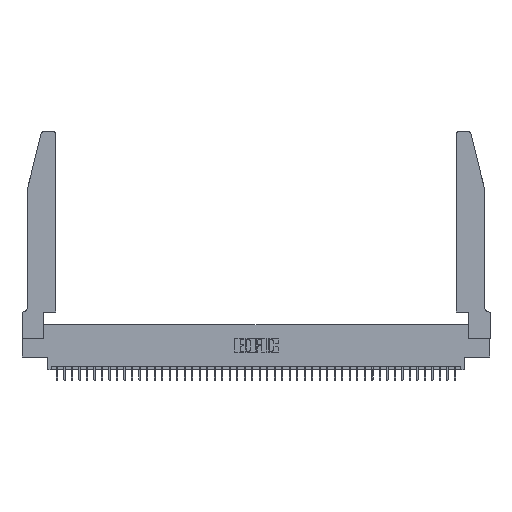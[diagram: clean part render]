
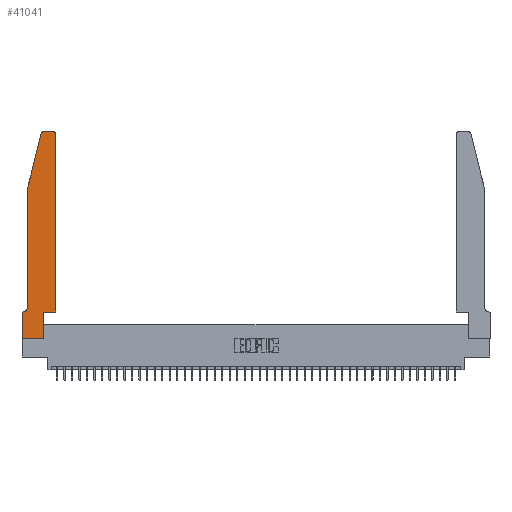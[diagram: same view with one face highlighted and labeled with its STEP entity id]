
A CAD part, top view. The second image highlights one B-rep face of the part: STEP entity #41041.
In plain terms, the highlighted planar face has unit normal (0, 0, 1).
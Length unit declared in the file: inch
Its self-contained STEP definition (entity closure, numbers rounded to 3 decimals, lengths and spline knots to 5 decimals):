
#462 = VECTOR ( 'NONE', #35885, 39.37008 ) ;
#1172 = CARTESIAN_POINT ( 'NONE',  ( 0., 0., 0.37 ) ) ;
#1195 = AXIS2_PLACEMENT_3D ( 'NONE', #23388, #37532, #28469 ) ;
#1721 = DIRECTION ( 'NONE',  ( 0., 1., 0. ) ) ;
#1767 = DIRECTION ( 'NONE',  ( 1., 0., 0. ) ) ;
#1785 = CARTESIAN_POINT ( 'NONE',  ( 0.4505, 0.35, 0.37 ) ) ;
#2930 = DIRECTION ( 'NONE',  ( 1., 0., 0. ) ) ;
#3050 = VERTEX_POINT ( 'NONE', #35194 ) ;
#3228 = ORIENTED_EDGE ( 'NONE', *, *, #13196, .T. ) ;
#3645 = ORIENTED_EDGE ( 'NONE', *, *, #19664, .T. ) ;
#3916 = VERTEX_POINT ( 'NONE', #27930 ) ;
#4370 = DIRECTION ( 'NONE',  ( 1., 0., 0. ) ) ;
#4557 = DIRECTION ( 'NONE',  ( -1., 0., 0. ) ) ;
#4720 = CARTESIAN_POINT ( 'NONE',  ( 0.2865, 0.35, 0.37 ) ) ;
#4751 = CARTESIAN_POINT ( 'NONE',  ( 0.284, 2.75, 0.37 ) ) ;
#5192 = CARTESIAN_POINT ( 'NONE',  ( 0.4505, 0.35, 0.37 ) ) ;
#5408 = EDGE_CURVE ( 'NONE', #26392, #32758, #25378, .T. ) ;
#6141 = FACE_OUTER_BOUND ( 'NONE', #27769, .T. ) ;
#6205 = AXIS2_PLACEMENT_3D ( 'NONE', #40865, #34358, #19552 ) ;
#6718 = EDGE_CURVE ( 'NONE', #16351, #27173, #20838, .T. ) ;
#7809 = CARTESIAN_POINT ( 'NONE',  ( 0.25487, 2.72718, 0.37 ) ) ;
#9042 = EDGE_CURVE ( 'NONE', #11569, #45186, #36239, .T. ) ;
#9110 = AXIS2_PLACEMENT_3D ( 'NONE', #21415, #35545, #1767 ) ;
#10266 = ORIENTED_EDGE ( 'NONE', *, *, #12650, .T. ) ;
#10383 = VERTEX_POINT ( 'NONE', #24129 ) ;
#11528 = CARTESIAN_POINT ( 'NONE',  ( 0., 0., 0.37 ) ) ;
#11569 = VERTEX_POINT ( 'NONE', #38325 ) ;
#11665 = LINE ( 'NONE', #5192, #41774 ) ;
#12535 = ORIENTED_EDGE ( 'NONE', *, *, #34317, .T. ) ;
#12650 = EDGE_CURVE ( 'NONE', #10383, #20875, #21471, .T. ) ;
#12747 = CARTESIAN_POINT ( 'NONE',  ( 0., 0.35, 0.37 ) ) ;
#13086 = EDGE_CURVE ( 'NONE', #27173, #13554, #29068, .T. ) ;
#13196 = EDGE_CURVE ( 'NONE', #3916, #26392, #24596, .T. ) ;
#13554 = VERTEX_POINT ( 'NONE', #31784 ) ;
#13767 = VERTEX_POINT ( 'NONE', #4720 ) ;
#13777 = VECTOR ( 'NONE', #44346, 39.37008 ) ;
#13927 = AXIS2_PLACEMENT_3D ( 'NONE', #45055, #27450, #2930 ) ;
#14813 = ORIENTED_EDGE ( 'NONE', *, *, #6718, .T. ) ;
#16254 = ORIENTED_EDGE ( 'NONE', *, *, #13086, .T. ) ;
#16351 = VERTEX_POINT ( 'NONE', #7809 ) ;
#18314 = VECTOR ( 'NONE', #4557, 39.37008 ) ;
#18804 = CARTESIAN_POINT ( 'NONE',  ( 0.2865, 0., 0.37 ) ) ;
#19552 = DIRECTION ( 'NONE',  ( 1., 0., 0. ) ) ;
#19664 = EDGE_CURVE ( 'NONE', #45186, #10383, #43739, .T. ) ;
#20245 = PLANE ( 'NONE',  #6205 ) ;
#20792 = CARTESIAN_POINT ( 'NONE',  ( 0.4205, 2.75, 0.37 ) ) ;
#20838 = LINE ( 'NONE', #31484, #462 ) ;
#20875 = VERTEX_POINT ( 'NONE', #18804 ) ;
#21415 = CARTESIAN_POINT ( 'NONE',  ( 0.4205, 2.72, 0.37 ) ) ;
#21471 = LINE ( 'NONE', #11528, #40866 ) ;
#22107 = CARTESIAN_POINT ( 'NONE',  ( 0.0755, 2., 0.37 ) ) ;
#22359 = LINE ( 'NONE', #1785, #13777 ) ;
#23388 = CARTESIAN_POINT ( 'NONE',  ( 0.0055, 0.42, 0.37 ) ) ;
#24129 = CARTESIAN_POINT ( 'NONE',  ( 0., 0., 0.37 ) ) ;
#24596 = CIRCLE ( 'NONE', #9110, 0.03 ) ;
#25378 = LINE ( 'NONE', #36483, #26999 ) ;
#25459 = ORIENTED_EDGE ( 'NONE', *, *, #28921, .T. ) ;
#26392 = VERTEX_POINT ( 'NONE', #20792 ) ;
#26472 = ORIENTED_EDGE ( 'NONE', *, *, #35015, .T. ) ;
#26486 = CIRCLE ( 'NONE', #13927, 0.03 ) ;
#26999 = VECTOR ( 'NONE', #39284, 39.37008 ) ;
#27173 = VERTEX_POINT ( 'NONE', #22107 ) ;
#27450 = DIRECTION ( 'NONE',  ( 0., 0., 1. ) ) ;
#27769 = EDGE_LOOP ( 'NONE', ( #30589, #12535, #14813, #16254, #40771, #35843, #3645, #10266, #26472, #34565, #25459, #3228 ) ) ;
#27930 = CARTESIAN_POINT ( 'NONE',  ( 0.4505, 2.72, 0.37 ) ) ;
#28469 = DIRECTION ( 'NONE',  ( -1., 0., 0. ) ) ;
#28510 = CARTESIAN_POINT ( 'NONE',  ( 0.2865, 0.35, 0.37 ) ) ;
#28842 = DIRECTION ( 'NONE',  ( 0., -1., 0. ) ) ;
#28921 = EDGE_CURVE ( 'NONE', #3050, #3916, #11665, .T. ) ;
#29068 = LINE ( 'NONE', #35313, #38718 ) ;
#29533 = EDGE_CURVE ( 'NONE', #13554, #11569, #41815, .T. ) ;
#30589 = ORIENTED_EDGE ( 'NONE', *, *, #5408, .T. ) ;
#31484 = CARTESIAN_POINT ( 'NONE',  ( 0.0755, 2., 0.37 ) ) ;
#31784 = CARTESIAN_POINT ( 'NONE',  ( 0.0755, 0.42, 0.37 ) ) ;
#32758 = VERTEX_POINT ( 'NONE', #4751 ) ;
#33323 = DIRECTION ( 'NONE',  ( 0., -1., 0. ) ) ;
#33931 = VECTOR ( 'NONE', #43291, 39.37008 ) ;
#34317 = EDGE_CURVE ( 'NONE', #32758, #16351, #26486, .T. ) ;
#34358 = DIRECTION ( 'NONE',  ( 0., 0., 1. ) ) ;
#34565 = ORIENTED_EDGE ( 'NONE', *, *, #42759, .T. ) ;
#34722 = VECTOR ( 'NONE', #33323, 39.37008 ) ;
#35015 = EDGE_CURVE ( 'NONE', #20875, #13767, #40080, .T. ) ;
#35194 = CARTESIAN_POINT ( 'NONE',  ( 0.4505, 0.35, 0.37 ) ) ;
#35313 = CARTESIAN_POINT ( 'NONE',  ( 0.0755, 2., 0.37 ) ) ;
#35545 = DIRECTION ( 'NONE',  ( 0., 0., 1. ) ) ;
#35843 = ORIENTED_EDGE ( 'NONE', *, *, #9042, .T. ) ;
#35885 = DIRECTION ( 'NONE',  ( -0.239, -0.971, 0. ) ) ;
#36008 = CARTESIAN_POINT ( 'NONE',  ( 0.0755, 0.35, 0.37 ) ) ;
#36239 = LINE ( 'NONE', #36008, #18314 ) ;
#36483 = CARTESIAN_POINT ( 'NONE',  ( 0.2605, 2.75, 0.37 ) ) ;
#37532 = DIRECTION ( 'NONE',  ( 0., 0., -1. ) ) ;
#38325 = CARTESIAN_POINT ( 'NONE',  ( 0.0055, 0.35, 0.37 ) ) ;
#38718 = VECTOR ( 'NONE', #28842, 39.37008 ) ;
#39284 = DIRECTION ( 'NONE',  ( -1., 0., 0. ) ) ;
#40080 = LINE ( 'NONE', #28510, #33931 ) ;
#40771 = ORIENTED_EDGE ( 'NONE', *, *, #29533, .T. ) ;
#40865 = CARTESIAN_POINT ( 'NONE',  ( 0., 0.35, 0.37 ) ) ;
#40866 = VECTOR ( 'NONE', #4370, 39.37008 ) ;
#41041 = ADVANCED_FACE ( 'NONE', ( #6141 ), #20245, .T. ) ;
#41774 = VECTOR ( 'NONE', #1721, 39.37008 ) ;
#41815 = CIRCLE ( 'NONE', #1195, 0.07 ) ;
#42759 = EDGE_CURVE ( 'NONE', #13767, #3050, #22359, .T. ) ;
#43291 = DIRECTION ( 'NONE',  ( 0., 1., 0. ) ) ;
#43739 = LINE ( 'NONE', #1172, #34722 ) ;
#44346 = DIRECTION ( 'NONE',  ( 1., 0., 0. ) ) ;
#45055 = CARTESIAN_POINT ( 'NONE',  ( 0.284, 2.72, 0.37 ) ) ;
#45186 = VERTEX_POINT ( 'NONE', #12747 ) ;
